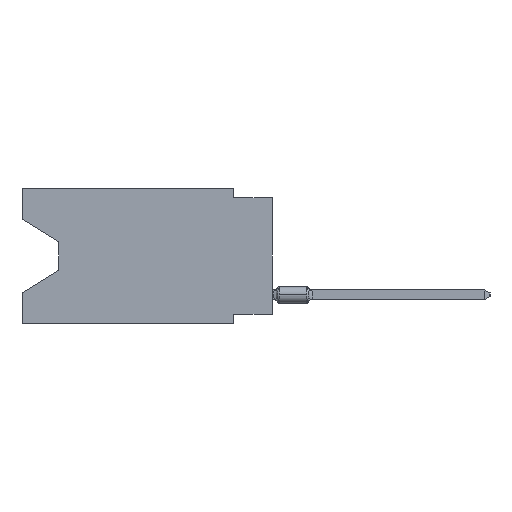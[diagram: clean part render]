
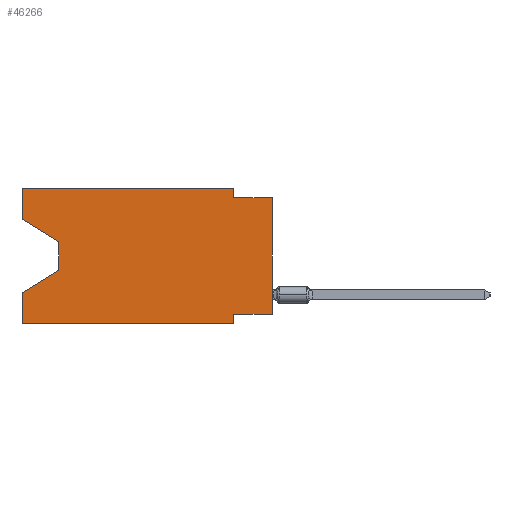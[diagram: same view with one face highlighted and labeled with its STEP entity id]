
A CAD part, left-side view. The second image highlights one B-rep face of the part: STEP entity #46266.
In plain terms, the highlighted planar face has unit normal (-1, 0, 0).
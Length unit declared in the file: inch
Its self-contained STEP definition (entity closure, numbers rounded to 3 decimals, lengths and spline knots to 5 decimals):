
#556 = EDGE_CURVE ( 'NONE', #47441, #4089, #16601, .T. ) ;
#748 = CARTESIAN_POINT ( 'NONE',  ( 0., 0., 0. ) ) ;
#786 = CARTESIAN_POINT ( 'NONE',  ( 0., 0.645, -0.35 ) ) ;
#966 = ORIENTED_EDGE ( 'NONE', *, *, #38487, .F. ) ;
#1170 = CARTESIAN_POINT ( 'NONE',  ( 0., 0.1, -0.35 ) ) ;
#1517 = DIRECTION ( 'NONE',  ( 0., 0.855, -0.519 ) ) ;
#2134 = VECTOR ( 'NONE', #44472, 39.37008 ) ;
#2192 = CARTESIAN_POINT ( 'NONE',  ( 0., 0.1, 0. ) ) ;
#2578 = LINE ( 'NONE', #22012, #35425 ) ;
#4089 = VERTEX_POINT ( 'NONE', #18818 ) ;
#4179 = EDGE_CURVE ( 'NONE', #20766, #36971, #35448, .T. ) ;
#5047 = DIRECTION ( 'NONE',  ( 0., 0., -1. ) ) ;
#5551 = ORIENTED_EDGE ( 'NONE', *, *, #34198, .F. ) ;
#6246 = CARTESIAN_POINT ( 'NONE',  ( 0., 0.645, -0.08025 ) ) ;
#6266 = EDGE_CURVE ( 'NONE', #29879, #40174, #20401, .T. ) ;
#6394 = DIRECTION ( 'NONE',  ( 0., 0., 1. ) ) ;
#8086 = DIRECTION ( 'NONE',  ( 0., -0.855, -0.519 ) ) ;
#8278 = VECTOR ( 'NONE', #1517, 39.37008 ) ;
#8454 = EDGE_CURVE ( 'NONE', #9880, #10686, #41809, .T. ) ;
#9632 = AXIS2_PLACEMENT_3D ( 'NONE', #48058, #40096, #5047 ) ;
#9880 = VERTEX_POINT ( 'NONE', #786 ) ;
#9976 = EDGE_CURVE ( 'NONE', #36971, #47441, #22465, .T. ) ;
#10567 = ORIENTED_EDGE ( 'NONE', *, *, #556, .T. ) ;
#10686 = VERTEX_POINT ( 'NONE', #1170 ) ;
#12423 = CARTESIAN_POINT ( 'NONE',  ( 0., 0.645, -0.08025 ) ) ;
#12594 = CARTESIAN_POINT ( 'NONE',  ( 0., 0., -0.025 ) ) ;
#12914 = EDGE_CURVE ( 'NONE', #33766, #29879, #38449, .T. ) ;
#13082 = ORIENTED_EDGE ( 'NONE', *, *, #6266, .F. ) ;
#13346 = VERTEX_POINT ( 'NONE', #43128 ) ;
#14417 = CARTESIAN_POINT ( 'NONE',  ( 0., 0., -0.325 ) ) ;
#14634 = CARTESIAN_POINT ( 'NONE',  ( 0., 0.645, 0. ) ) ;
#16601 = LINE ( 'NONE', #32200, #8278 ) ;
#16855 = VECTOR ( 'NONE', #41466, 39.37008 ) ;
#17145 = LINE ( 'NONE', #32738, #43566 ) ;
#17779 = DIRECTION ( 'NONE',  ( 0., 0., -1. ) ) ;
#18818 = CARTESIAN_POINT ( 'NONE',  ( 0., 0.645, -0.26975 ) ) ;
#20401 = LINE ( 'NONE', #2192, #33933 ) ;
#20766 = VERTEX_POINT ( 'NONE', #6246 ) ;
#22012 = CARTESIAN_POINT ( 'NONE',  ( 0., 0., -0.025 ) ) ;
#22339 = CARTESIAN_POINT ( 'NONE',  ( 0., 0.55, -0.212 ) ) ;
#22357 = CARTESIAN_POINT ( 'NONE',  ( 0., 0.645, -0.35 ) ) ;
#22465 = LINE ( 'NONE', #33251, #27921 ) ;
#23520 = ORIENTED_EDGE ( 'NONE', *, *, #49721, .T. ) ;
#24092 = VERTEX_POINT ( 'NONE', #12594 ) ;
#24471 = PLANE ( 'NONE',  #9632 ) ;
#25013 = VERTEX_POINT ( 'NONE', #30127 ) ;
#25779 = VECTOR ( 'NONE', #8086, 39.37008 ) ;
#25831 = DIRECTION ( 'NONE',  ( 0., 0., -1. ) ) ;
#25861 = LINE ( 'NONE', #49151, #16855 ) ;
#26450 = DIRECTION ( 'NONE',  ( 0., -1., 0. ) ) ;
#26695 = VECTOR ( 'NONE', #34160, 39.37008 ) ;
#27053 = ORIENTED_EDGE ( 'NONE', *, *, #9976, .T. ) ;
#27517 = CARTESIAN_POINT ( 'NONE',  ( 0., 0.645, 0. ) ) ;
#27614 = ORIENTED_EDGE ( 'NONE', *, *, #12914, .F. ) ;
#27921 = VECTOR ( 'NONE', #25831, 39.37008 ) ;
#28777 = CARTESIAN_POINT ( 'NONE',  ( 0., 0.1, -0.025 ) ) ;
#28852 = LINE ( 'NONE', #748, #2134 ) ;
#29740 = EDGE_CURVE ( 'NONE', #40174, #24092, #2578, .T. ) ;
#29879 = VERTEX_POINT ( 'NONE', #42975 ) ;
#30019 = DIRECTION ( 'NONE',  ( 0., 1., 0. ) ) ;
#30127 = CARTESIAN_POINT ( 'NONE',  ( 0., 0.1, -0.325 ) ) ;
#31077 = LINE ( 'NONE', #27517, #26695 ) ;
#31834 = CARTESIAN_POINT ( 'NONE',  ( 0., 0.55, -0.138 ) ) ;
#32200 = CARTESIAN_POINT ( 'NONE',  ( 0., 0.55, -0.212 ) ) ;
#32738 = CARTESIAN_POINT ( 'NONE',  ( 0., 0.645, 0. ) ) ;
#32896 = VECTOR ( 'NONE', #26450, 39.37008 ) ;
#33251 = CARTESIAN_POINT ( 'NONE',  ( 0., 0.55, -0.138 ) ) ;
#33766 = VERTEX_POINT ( 'NONE', #14634 ) ;
#33933 = VECTOR ( 'NONE', #17779, 39.37008 ) ;
#34160 = DIRECTION ( 'NONE',  ( 0., 0., 1. ) ) ;
#34198 = EDGE_CURVE ( 'NONE', #25013, #10686, #25861, .T. ) ;
#35425 = VECTOR ( 'NONE', #45311, 39.37008 ) ;
#35448 = LINE ( 'NONE', #12423, #25779 ) ;
#35982 = ORIENTED_EDGE ( 'NONE', *, *, #8454, .T. ) ;
#36137 = VECTOR ( 'NONE', #30019, 39.37008 ) ;
#36507 = FACE_OUTER_BOUND ( 'NONE', #43895, .T. ) ;
#36971 = VERTEX_POINT ( 'NONE', #31834 ) ;
#38215 = CARTESIAN_POINT ( 'NONE',  ( 0., 0.645, 0. ) ) ;
#38449 = LINE ( 'NONE', #38215, #32896 ) ;
#38487 = EDGE_CURVE ( 'NONE', #13346, #25013, #49489, .T. ) ;
#39412 = ORIENTED_EDGE ( 'NONE', *, *, #4179, .T. ) ;
#39956 = ORIENTED_EDGE ( 'NONE', *, *, #45349, .F. ) ;
#40096 = DIRECTION ( 'NONE',  ( 1., 0., 0. ) ) ;
#40174 = VERTEX_POINT ( 'NONE', #28777 ) ;
#41199 = EDGE_CURVE ( 'NONE', #9880, #4089, #17145, .T. ) ;
#41276 = ORIENTED_EDGE ( 'NONE', *, *, #41199, .F. ) ;
#41466 = DIRECTION ( 'NONE',  ( 0., 0., -1. ) ) ;
#41809 = LINE ( 'NONE', #22357, #49048 ) ;
#42975 = CARTESIAN_POINT ( 'NONE',  ( 0., 0.1, 0. ) ) ;
#43128 = CARTESIAN_POINT ( 'NONE',  ( 0., 0., -0.325 ) ) ;
#43566 = VECTOR ( 'NONE', #6394, 39.37008 ) ;
#43895 = EDGE_LOOP ( 'NONE', ( #39412, #27053, #10567, #41276, #35982, #5551, #966, #23520, #44766, #13082, #27614, #39956 ) ) ;
#44472 = DIRECTION ( 'NONE',  ( 0., 0., 1. ) ) ;
#44766 = ORIENTED_EDGE ( 'NONE', *, *, #29740, .F. ) ;
#45311 = DIRECTION ( 'NONE',  ( 0., -1., 0. ) ) ;
#45349 = EDGE_CURVE ( 'NONE', #20766, #33766, #31077, .T. ) ;
#46266 = ADVANCED_FACE ( 'NONE', ( #36507 ), #24471, .F. ) ;
#47441 = VERTEX_POINT ( 'NONE', #22339 ) ;
#48058 = CARTESIAN_POINT ( 'NONE',  ( 0., 0.645, 0. ) ) ;
#49048 = VECTOR ( 'NONE', #50012, 39.37008 ) ;
#49151 = CARTESIAN_POINT ( 'NONE',  ( 0., 0.1, -0.35 ) ) ;
#49489 = LINE ( 'NONE', #14417, #36137 ) ;
#49721 = EDGE_CURVE ( 'NONE', #13346, #24092, #28852, .T. ) ;
#50012 = DIRECTION ( 'NONE',  ( 0., -1., 0. ) ) ;
